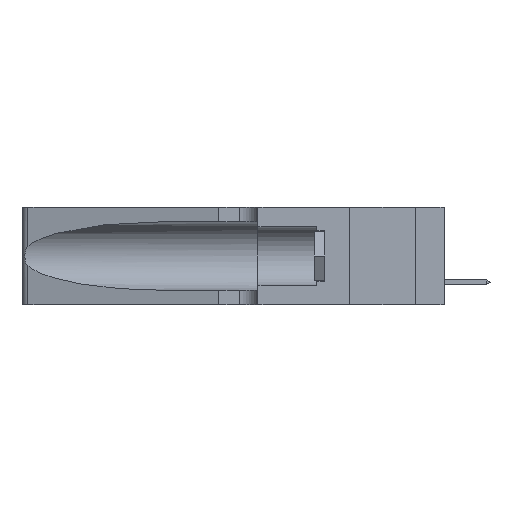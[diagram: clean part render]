
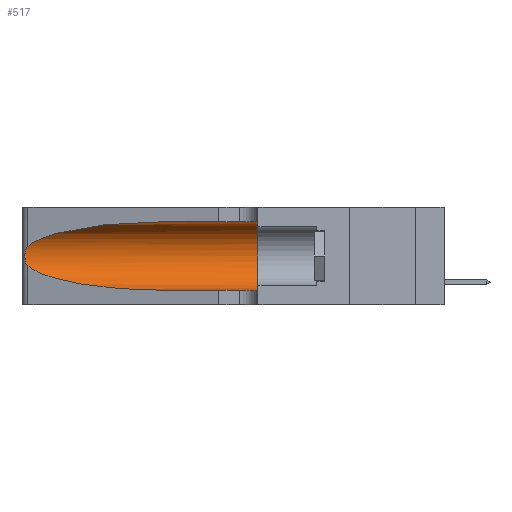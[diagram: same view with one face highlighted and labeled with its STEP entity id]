
A CAD part, left-side view. The second image highlights one B-rep face of the part: STEP entity #517.
In plain terms, the highlighted cylindrical face has radius 3.308 mm (diameter 6.617 mm), a partial arc.
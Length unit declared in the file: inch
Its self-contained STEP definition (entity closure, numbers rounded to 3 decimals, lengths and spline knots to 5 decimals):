
#30 = DIRECTION ( 'NONE',  ( 0., 1., 0. ) ) ;
#441 = CARTESIAN_POINT ( 'NONE',  ( 0.25487, 1.22718, 0.22369 ) ) ;
#517 = ADVANCED_FACE ( 'NONE', ( #10518 ), #3987, .F. ) ;
#685 = CARTESIAN_POINT ( 'NONE',  ( 0.25555, 1.22993, 0.14849 ) ) ;
#811 = CARTESIAN_POINT ( 'NONE',  ( 0.1305, 0.35, 0.05475 ) ) ;
#1934 = EDGE_CURVE ( 'NONE', #21047, #11389, #7453, .T. ) ;
#1952 = CARTESIAN_POINT ( 'NONE',  ( 0.25854, 1.2359, 0.20912 ) ) ;
#2514 = EDGE_CURVE ( 'NONE', #8463, #11389, #15298, .T. ) ;
#2527 = CARTESIAN_POINT ( 'NONE',  ( 0.2373, 1.15595, 0.28018 ) ) ;
#2629 = VECTOR ( 'NONE', #5383, 39.37008 ) ;
#3386 =( BOUNDED_CURVE ( )  B_SPLINE_CURVE ( 3, ( #5790, #11173, #19842, #3940 ),
 .UNSPECIFIED., .F., .T. ) 
 B_SPLINE_CURVE_WITH_KNOTS ( ( 4, 4 ),
 ( 3.44316, 4.71239 ),
 .UNSPECIFIED. ) 
 CURVE ( )  GEOMETRIC_REPRESENTATION_ITEM ( )  RATIONAL_B_SPLINE_CURVE ( ( 1., 0.87, 0.87, 1. ) ) 
 REPRESENTATION_ITEM ( '' )  );
#3940 = CARTESIAN_POINT ( 'NONE',  ( 0.1305, 0.72297, 0.05475 ) ) ;
#3987 = CYLINDRICAL_SURFACE ( 'NONE', #19409, 0.13025 ) ;
#5383 = DIRECTION ( 'NONE',  ( 0., -1., 0. ) ) ;
#5719 = CARTESIAN_POINT ( 'NONE',  ( 0.25789, 1.23486, 0.15765 ) ) ;
#5790 = CARTESIAN_POINT ( 'NONE',  ( 0.25487, 1.22718, 0.14631 ) ) ;
#6022 = CARTESIAN_POINT ( 'NONE',  ( 0.26075, 1.23896, 0.19203 ) ) ;
#6583 = CARTESIAN_POINT ( 'NONE',  ( 0.1305, 0.72297, 0.05475 ) ) ;
#7453 = LINE ( 'NONE', #13217, #12859 ) ;
#7905 = EDGE_CURVE ( 'NONE', #14743, #8463, #9392, .T. ) ;
#7922 = CARTESIAN_POINT ( 'NONE',  ( 0.25487, 1.22718, 0.22369 ) ) ;
#8169 = CARTESIAN_POINT ( 'NONE',  ( 0.1305, 1.61858, 0.185 ) ) ;
#8463 = VERTEX_POINT ( 'NONE', #10757 ) ;
#8963 = EDGE_CURVE ( 'NONE', #13098, #20741, #12418, .T. ) ;
#9104 = CARTESIAN_POINT ( 'NONE',  ( 0.25487, 1.22718, 0.22369 ) ) ;
#9369 =( BOUNDED_CURVE ( )  B_SPLINE_CURVE ( 3, ( #21305, #18205, #2527, #7922 ),
 .UNSPECIFIED., .F., .F. ) 
 B_SPLINE_CURVE_WITH_KNOTS ( ( 4, 4 ),
 ( 1.5708, 2.84003 ),
 .UNSPECIFIED. ) 
 CURVE ( )  GEOMETRIC_REPRESENTATION_ITEM ( )  RATIONAL_B_SPLINE_CURVE ( ( 1., 0.87, 0.87, 1. ) ) 
 REPRESENTATION_ITEM ( '' )  );
#9392 = LINE ( 'NONE', #14150, #2629 ) ;
#9574 = ORIENTED_EDGE ( 'NONE', *, *, #18297, .T. ) ;
#10518 = FACE_OUTER_BOUND ( 'NONE', #16688, .T. ) ;
#10572 = CARTESIAN_POINT ( 'NONE',  ( 0.25639, 1.23184, 0.21858 ) ) ;
#10757 = CARTESIAN_POINT ( 'NONE',  ( 0.1305, 0.35, 0.31525 ) ) ;
#10873 = CARTESIAN_POINT ( 'NONE',  ( 0.26017, 1.23833, 0.17102 ) ) ;
#11173 = CARTESIAN_POINT ( 'NONE',  ( 0.2373, 1.15595, 0.08982 ) ) ;
#11174 = CARTESIAN_POINT ( 'NONE',  ( 0.25856, 1.23593, 0.16098 ) ) ;
#11262 = ORIENTED_EDGE ( 'NONE', *, *, #8963, .T. ) ;
#11389 = VERTEX_POINT ( 'NONE', #811 ) ;
#11621 = DIRECTION ( 'NONE',  ( 0., -1., 0. ) ) ;
#12298 = CARTESIAN_POINT ( 'NONE',  ( 0.25787, 1.23484, 0.2124 ) ) ;
#12418 = B_SPLINE_CURVE_WITH_KNOTS ( 'NONE', 3,
 ( #9104, #15707, #10572, #12298, #1952, #14111, #6022, #14657, #10873, #11174, #5719, #21382, #685, #21228 ),
 .UNSPECIFIED., .F., .F.,
 ( 4, 2, 2, 2, 2, 2, 4 ),
 ( 0., 0.00027, 0.00053, 0.00107, 0.0016, 0.00187, 0.00214 ),
 .UNSPECIFIED. ) ;
#12859 = VECTOR ( 'NONE', #11621, 39.37008 ) ;
#13098 = VERTEX_POINT ( 'NONE', #441 ) ;
#13217 = CARTESIAN_POINT ( 'NONE',  ( 0.1305, 1.61858, 0.05475 ) ) ;
#14111 = CARTESIAN_POINT ( 'NONE',  ( 0.26018, 1.23835, 0.19895 ) ) ;
#14150 = CARTESIAN_POINT ( 'NONE',  ( 0.1305, 1.61858, 0.31525 ) ) ;
#14657 = CARTESIAN_POINT ( 'NONE',  ( 0.26075, 1.23896, 0.178 ) ) ;
#14695 = ORIENTED_EDGE ( 'NONE', *, *, #7905, .F. ) ;
#14743 = VERTEX_POINT ( 'NONE', #15671 ) ;
#15298 = CIRCLE ( 'NONE', #17003, 0.13025 ) ;
#15484 = DIRECTION ( 'NONE',  ( 0., -1., 0. ) ) ;
#15671 = CARTESIAN_POINT ( 'NONE',  ( 0.1305, 0.72297, 0.31525 ) ) ;
#15707 = CARTESIAN_POINT ( 'NONE',  ( 0.25555, 1.22994, 0.2215 ) ) ;
#16461 = ORIENTED_EDGE ( 'NONE', *, *, #1934, .T. ) ;
#16688 = EDGE_LOOP ( 'NONE', ( #9574, #11262, #17393, #16461, #19410, #14695 ) ) ;
#17003 = AXIS2_PLACEMENT_3D ( 'NONE', #18879, #30, #20720 ) ;
#17363 = DIRECTION ( 'NONE',  ( 0., 0., -1. ) ) ;
#17393 = ORIENTED_EDGE ( 'NONE', *, *, #21528, .T. ) ;
#18205 = CARTESIAN_POINT ( 'NONE',  ( 0.18966, 0.96281, 0.31525 ) ) ;
#18297 = EDGE_CURVE ( 'NONE', #14743, #13098, #9369, .T. ) ;
#18879 = CARTESIAN_POINT ( 'NONE',  ( 0.1305, 0.35, 0.185 ) ) ;
#19052 = CARTESIAN_POINT ( 'NONE',  ( 0.25487, 1.22718, 0.14631 ) ) ;
#19409 = AXIS2_PLACEMENT_3D ( 'NONE', #8169, #15484, #17363 ) ;
#19410 = ORIENTED_EDGE ( 'NONE', *, *, #2514, .F. ) ;
#19842 = CARTESIAN_POINT ( 'NONE',  ( 0.18966, 0.96281, 0.05475 ) ) ;
#20720 = DIRECTION ( 'NONE',  ( 0., 0., 1. ) ) ;
#20741 = VERTEX_POINT ( 'NONE', #19052 ) ;
#21047 = VERTEX_POINT ( 'NONE', #6583 ) ;
#21228 = CARTESIAN_POINT ( 'NONE',  ( 0.25487, 1.22718, 0.14631 ) ) ;
#21305 = CARTESIAN_POINT ( 'NONE',  ( 0.1305, 0.72297, 0.31525 ) ) ;
#21382 = CARTESIAN_POINT ( 'NONE',  ( 0.25639, 1.23186, 0.15144 ) ) ;
#21528 = EDGE_CURVE ( 'NONE', #20741, #21047, #3386, .T. ) ;
